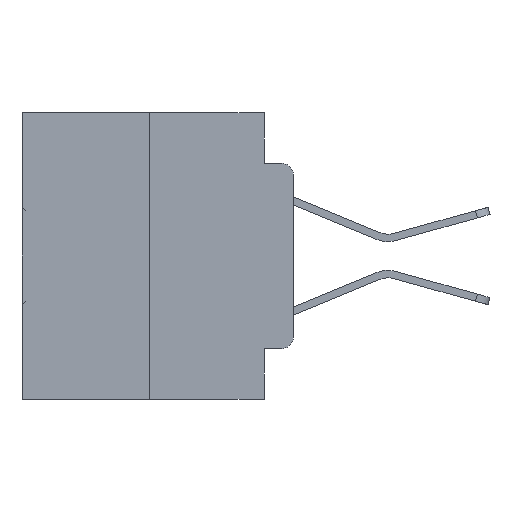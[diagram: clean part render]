
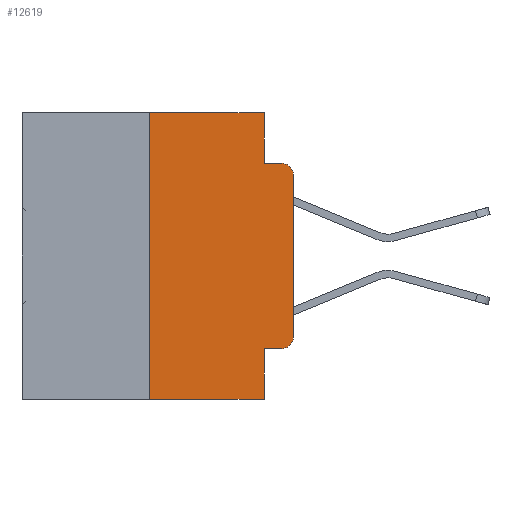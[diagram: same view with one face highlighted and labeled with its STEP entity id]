
A CAD part, left-side view. The second image highlights one B-rep face of the part: STEP entity #12619.
In plain terms, the highlighted planar face has unit normal (-1, 0, 0).
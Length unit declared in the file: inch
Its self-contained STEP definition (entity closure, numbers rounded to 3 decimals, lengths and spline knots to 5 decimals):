
#49 = LINE ( 'NONE', #15520, #10608 ) ;
#480 = DIRECTION ( 'NONE',  ( 0., -1., 0. ) ) ;
#708 = VECTOR ( 'NONE', #16876, 39.37008 ) ;
#2232 = CARTESIAN_POINT ( 'NONE',  ( 0., 0.02, -0.1085 ) ) ;
#2432 = DIRECTION ( 'NONE',  ( 1., 0., 0. ) ) ;
#3074 = CARTESIAN_POINT ( 'NONE',  ( 0., 0.473, 0. ) ) ;
#3385 = VECTOR ( 'NONE', #15357, 39.37008 ) ;
#3551 = VECTOR ( 'NONE', #6934, 39.37008 ) ;
#3712 = CARTESIAN_POINT ( 'NONE',  ( 0., 0.051, -0.5 ) ) ;
#4296 = CARTESIAN_POINT ( 'NONE',  ( 0., 0.051, -0.4115 ) ) ;
#5419 = DIRECTION ( 'NONE',  ( 0., 0., -1. ) ) ;
#5584 = DIRECTION ( 'NONE',  ( 0., -1., 0. ) ) ;
#5682 = DIRECTION ( 'NONE',  ( 0., 0., -1. ) ) ;
#5735 = VERTEX_POINT ( 'NONE', #12739 ) ;
#6934 = DIRECTION ( 'NONE',  ( 0., 0., 1. ) ) ;
#7619 = DIRECTION ( 'NONE',  ( -1., 0., 0. ) ) ;
#7774 = LINE ( 'NONE', #32922, #3385 ) ;
#7813 = PLANE ( 'NONE',  #20418 ) ;
#7949 = CARTESIAN_POINT ( 'NONE',  ( 0., 0.02, -0.4115 ) ) ;
#8341 = AXIS2_PLACEMENT_3D ( 'NONE', #31655, #31819, #5682 ) ;
#8687 = DIRECTION ( 'NONE',  ( 0., 0., -1. ) ) ;
#8957 = ORIENTED_EDGE ( 'NONE', *, *, #11334, .F. ) ;
#9068 = VERTEX_POINT ( 'NONE', #13350 ) ;
#9096 = ORIENTED_EDGE ( 'NONE', *, *, #27006, .F. ) ;
#9146 = LINE ( 'NONE', #32589, #708 ) ;
#9794 = VERTEX_POINT ( 'NONE', #7949 ) ;
#10030 = CARTESIAN_POINT ( 'NONE',  ( 0., 0.02, -0.0885 ) ) ;
#10283 = VERTEX_POINT ( 'NONE', #18057 ) ;
#10335 = FACE_OUTER_BOUND ( 'NONE', #18553, .T. ) ;
#10608 = VECTOR ( 'NONE', #5584, 39.37008 ) ;
#11334 = EDGE_CURVE ( 'NONE', #23966, #26356, #31948, .T. ) ;
#11891 = LINE ( 'NONE', #31808, #17574 ) ;
#12296 = VECTOR ( 'NONE', #480, 39.37008 ) ;
#12619 = ADVANCED_FACE ( 'NONE', ( #10335 ), #7813, .F. ) ;
#12739 = CARTESIAN_POINT ( 'NONE',  ( 0., 0.051, -0.4115 ) ) ;
#12808 = VERTEX_POINT ( 'NONE', #3712 ) ;
#13350 = CARTESIAN_POINT ( 'NONE',  ( 0., 0.051, 0. ) ) ;
#15357 = DIRECTION ( 'NONE',  ( 0., 0., -1. ) ) ;
#15520 = CARTESIAN_POINT ( 'NONE',  ( 0., 0.473, -0.5 ) ) ;
#16255 = VECTOR ( 'NONE', #17411, 39.37008 ) ;
#16290 = CARTESIAN_POINT ( 'NONE',  ( 0., 0., -0.1085 ) ) ;
#16397 = EDGE_CURVE ( 'NONE', #10283, #21559, #9146, .T. ) ;
#16453 = EDGE_CURVE ( 'NONE', #5735, #12808, #7774, .T. ) ;
#16876 = DIRECTION ( 'NONE',  ( 0., 0., 1. ) ) ;
#17073 = AXIS2_PLACEMENT_3D ( 'NONE', #2232, #7619, #5419 ) ;
#17411 = DIRECTION ( 'NONE',  ( 0., -1., 0. ) ) ;
#17574 = VECTOR ( 'NONE', #8687, 39.37008 ) ;
#17579 = CARTESIAN_POINT ( 'NONE',  ( 0., 0.473, 0. ) ) ;
#17720 = ORIENTED_EDGE ( 'NONE', *, *, #17719, .T. ) ;
#17719 = EDGE_CURVE ( 'NONE', #5735, #9794, #19613, .T. ) ;
#18057 = CARTESIAN_POINT ( 'NONE',  ( 0., 0.25, -0.5 ) ) ;
#18161 = CIRCLE ( 'NONE', #17073, 0.02 ) ;
#18553 = EDGE_LOOP ( 'NONE', ( #25142, #29160, #8957, #32996, #9096, #31302, #25543, #30810, #17720, #24534 ) ) ;
#19613 = LINE ( 'NONE', #4296, #16255 ) ;
#20418 = AXIS2_PLACEMENT_3D ( 'NONE', #17579, #2432, #22811 ) ;
#21230 = CARTESIAN_POINT ( 'NONE',  ( 0., 0., -0.3915 ) ) ;
#21559 = VERTEX_POINT ( 'NONE', #31400 ) ;
#21640 = CARTESIAN_POINT ( 'NONE',  ( 0., 0.051, -0.0885 ) ) ;
#22058 = EDGE_CURVE ( 'NONE', #9794, #32030, #33128, .T. ) ;
#22811 = DIRECTION ( 'NONE',  ( 0., 0., -1. ) ) ;
#23451 = DIRECTION ( 'NONE',  ( 0., -1., 0. ) ) ;
#23966 = VERTEX_POINT ( 'NONE', #21640 ) ;
#24534 = ORIENTED_EDGE ( 'NONE', *, *, #22058, .T. ) ;
#24965 = EDGE_CURVE ( 'NONE', #9068, #23966, #11891, .T. ) ;
#25142 = ORIENTED_EDGE ( 'NONE', *, *, #28602, .T. ) ;
#25543 = ORIENTED_EDGE ( 'NONE', *, *, #30724, .T. ) ;
#25620 = LINE ( 'NONE', #30046, #3551 ) ;
#26356 = VERTEX_POINT ( 'NONE', #10030 ) ;
#27006 = EDGE_CURVE ( 'NONE', #21559, #9068, #31572, .T. ) ;
#28602 = EDGE_CURVE ( 'NONE', #32030, #31169, #25620, .T. ) ;
#29160 = ORIENTED_EDGE ( 'NONE', *, *, #30690, .T. ) ;
#30046 = CARTESIAN_POINT ( 'NONE',  ( 0., 0., 0. ) ) ;
#30690 = EDGE_CURVE ( 'NONE', #31169, #26356, #18161, .T. ) ;
#30724 = EDGE_CURVE ( 'NONE', #10283, #12808, #49, .T. ) ;
#30810 = ORIENTED_EDGE ( 'NONE', *, *, #16453, .F. ) ;
#30986 = VECTOR ( 'NONE', #23451, 39.37008 ) ;
#31169 = VERTEX_POINT ( 'NONE', #16290 ) ;
#31302 = ORIENTED_EDGE ( 'NONE', *, *, #16397, .F. ) ;
#31400 = CARTESIAN_POINT ( 'NONE',  ( 0., 0.25, 0. ) ) ;
#31572 = LINE ( 'NONE', #3074, #30986 ) ;
#31655 = CARTESIAN_POINT ( 'NONE',  ( 0., 0.02, -0.3915 ) ) ;
#31808 = CARTESIAN_POINT ( 'NONE',  ( 0., 0.051, 0. ) ) ;
#31819 = DIRECTION ( 'NONE',  ( -1., 0., 0. ) ) ;
#31948 = LINE ( 'NONE', #32283, #12296 ) ;
#32030 = VERTEX_POINT ( 'NONE', #21230 ) ;
#32283 = CARTESIAN_POINT ( 'NONE',  ( 0., 0.051, -0.0885 ) ) ;
#32589 = CARTESIAN_POINT ( 'NONE',  ( 0., 0.25, 0. ) ) ;
#32922 = CARTESIAN_POINT ( 'NONE',  ( 0., 0.051, 0. ) ) ;
#32996 = ORIENTED_EDGE ( 'NONE', *, *, #24965, .F. ) ;
#33128 = CIRCLE ( 'NONE', #8341, 0.02 ) ;
